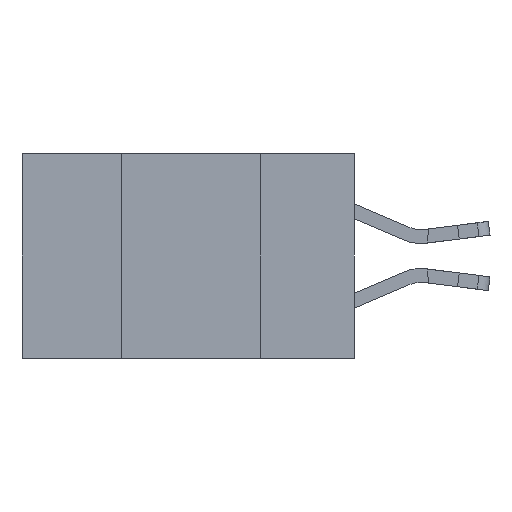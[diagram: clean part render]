
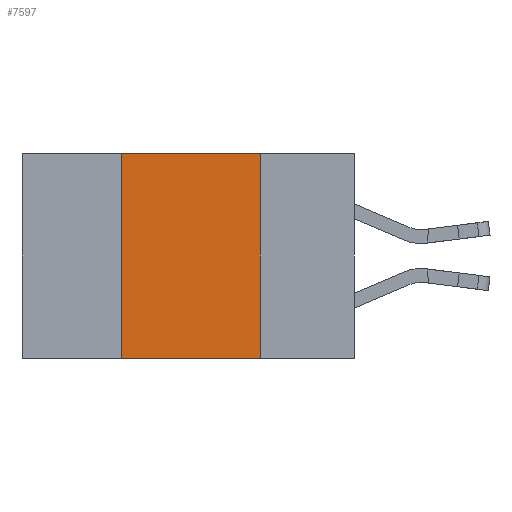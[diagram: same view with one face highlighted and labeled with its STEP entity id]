
A CAD part, left-side view. The second image highlights one B-rep face of the part: STEP entity #7597.
In plain terms, the highlighted planar face has unit normal (-1, 0, 0).
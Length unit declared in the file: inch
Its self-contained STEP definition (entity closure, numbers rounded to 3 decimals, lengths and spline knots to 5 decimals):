
#130 = AXIS2_PLACEMENT_3D ( 'NONE', #12749, #12455, #12437 ) ;
#1124 = CARTESIAN_POINT ( 'NONE',  ( 0., 0.17, -0.37 ) ) ;
#1700 = CARTESIAN_POINT ( 'NONE',  ( 0., 0.6, -0.37 ) ) ;
#1811 = CARTESIAN_POINT ( 'NONE',  ( 0., 0.6, 0. ) ) ;
#2349 = VERTEX_POINT ( 'NONE', #10633 ) ;
#4361 = EDGE_CURVE ( 'NONE', #2349, #22477, #19810, .T. ) ;
#4434 = DIRECTION ( 'NONE',  ( 0., 0., -1. ) ) ;
#4988 = CARTESIAN_POINT ( 'NONE',  ( 0., 0.17, 0. ) ) ;
#5684 = VECTOR ( 'NONE', #11646, 39.37008 ) ;
#6065 = EDGE_CURVE ( 'NONE', #9955, #10111, #17153, .T. ) ;
#6862 = LINE ( 'NONE', #1811, #12623 ) ;
#7293 = VECTOR ( 'NONE', #4434, 39.37008 ) ;
#7383 = DIRECTION ( 'NONE',  ( 0., -1., 0. ) ) ;
#7597 = ADVANCED_FACE ( 'NONE', ( #23240 ), #12703, .F. ) ;
#8020 = CARTESIAN_POINT ( 'NONE',  ( 0., 0.17, 0. ) ) ;
#9638 = EDGE_CURVE ( 'NONE', #22477, #9955, #6862, .T. ) ;
#9955 = VERTEX_POINT ( 'NONE', #8020 ) ;
#10060 = EDGE_LOOP ( 'NONE', ( #12271, #16986, #19153, #18544 ) ) ;
#10111 = VERTEX_POINT ( 'NONE', #1124 ) ;
#10633 = CARTESIAN_POINT ( 'NONE',  ( 0., 0.42, -0.37 ) ) ;
#10660 = VECTOR ( 'NONE', #10848, 39.37008 ) ;
#10848 = DIRECTION ( 'NONE',  ( 0., -1., 0. ) ) ;
#11646 = DIRECTION ( 'NONE',  ( 0., 0., 1. ) ) ;
#11986 = EDGE_CURVE ( 'NONE', #2349, #10111, #15235, .T. ) ;
#12271 = ORIENTED_EDGE ( 'NONE', *, *, #6065, .F. ) ;
#12437 = DIRECTION ( 'NONE',  ( 0., 0., -1. ) ) ;
#12455 = DIRECTION ( 'NONE',  ( 1., 0., 0. ) ) ;
#12623 = VECTOR ( 'NONE', #7383, 39.37008 ) ;
#12703 = PLANE ( 'NONE',  #130 ) ;
#12749 = CARTESIAN_POINT ( 'NONE',  ( 0., 0.6, 0. ) ) ;
#13146 = CARTESIAN_POINT ( 'NONE',  ( 0., 0.42, 0. ) ) ;
#15235 = LINE ( 'NONE', #1700, #10660 ) ;
#16986 = ORIENTED_EDGE ( 'NONE', *, *, #9638, .F. ) ;
#17153 = LINE ( 'NONE', #4988, #7293 ) ;
#17748 = CARTESIAN_POINT ( 'NONE',  ( 0., 0.42, 0. ) ) ;
#18544 = ORIENTED_EDGE ( 'NONE', *, *, #11986, .T. ) ;
#19153 = ORIENTED_EDGE ( 'NONE', *, *, #4361, .F. ) ;
#19810 = LINE ( 'NONE', #17748, #5684 ) ;
#22477 = VERTEX_POINT ( 'NONE', #13146 ) ;
#23240 = FACE_OUTER_BOUND ( 'NONE', #10060, .T. ) ;
